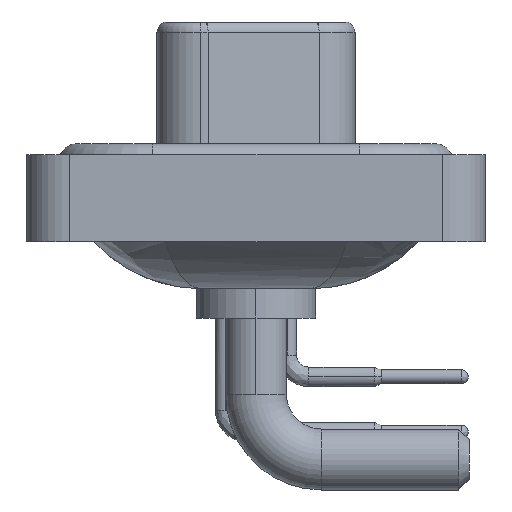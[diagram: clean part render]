
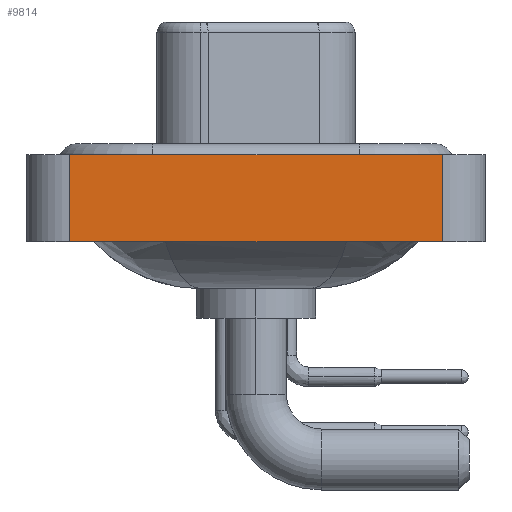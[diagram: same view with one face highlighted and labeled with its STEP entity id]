
A CAD part, left-side view. The second image highlights one B-rep face of the part: STEP entity #9814.
In plain terms, the highlighted planar face has unit normal (-1, 0, 0).
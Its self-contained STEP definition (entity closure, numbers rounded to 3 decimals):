
#1342 = CARTESIAN_POINT ( 'NONE',  ( -7.35, -8.55, 0.4 ) ) ;
#1466 = DIRECTION ( 'NONE',  ( 0., -1., 0. ) ) ;
#1738 = PLANE ( 'NONE',  #18898 ) ;
#3539 = DIRECTION ( 'NONE',  ( -1., 0., 0. ) ) ;
#3725 = EDGE_CURVE ( 'NONE', #19844, #24906, #16685, .T. ) ;
#3857 = DIRECTION ( 'NONE',  ( 0., 0., 1. ) ) ;
#4810 = ORIENTED_EDGE ( 'NONE', *, *, #3725, .F. ) ;
#5682 = CARTESIAN_POINT ( 'NONE',  ( -7.35, 8.55, -3.6 ) ) ;
#5730 = DIRECTION ( 'NONE',  ( 0., -1., 0. ) ) ;
#7687 = FACE_OUTER_BOUND ( 'NONE', #8082, .T. ) ;
#7811 = CARTESIAN_POINT ( 'NONE',  ( -7.35, -8.55, -3.6 ) ) ;
#8082 = EDGE_LOOP ( 'NONE', ( #26727, #4810, #15381, #11555 ) ) ;
#8461 = CARTESIAN_POINT ( 'NONE',  ( -7.35, -8.55, -3.6 ) ) ;
#9669 = VECTOR ( 'NONE', #24639, 1000. ) ;
#9814 = ADVANCED_FACE ( 'NONE', ( #7687 ), #1738, .T. ) ;
#10704 = EDGE_CURVE ( 'NONE', #17565, #19844, #15774, .T. ) ;
#11298 = EDGE_CURVE ( 'NONE', #12120, #24906, #16441, .T. ) ;
#11555 = ORIENTED_EDGE ( 'NONE', *, *, #19755, .T. ) ;
#12120 = VERTEX_POINT ( 'NONE', #8461 ) ;
#14320 = CARTESIAN_POINT ( 'NONE',  ( -7.35, -8.55, -3.6 ) ) ;
#15381 = ORIENTED_EDGE ( 'NONE', *, *, #10704, .F. ) ;
#15774 = LINE ( 'NONE', #5682, #9669 ) ;
#15986 = VECTOR ( 'NONE', #1466, 1000. ) ;
#16101 = LINE ( 'NONE', #7811, #23986 ) ;
#16441 = LINE ( 'NONE', #22824, #27150 ) ;
#16685 = LINE ( 'NONE', #20277, #15986 ) ;
#17565 = VERTEX_POINT ( 'NONE', #19744 ) ;
#18334 = CARTESIAN_POINT ( 'NONE',  ( -7.35, 8.55, 0.4 ) ) ;
#18898 = AXIS2_PLACEMENT_3D ( 'NONE', #14320, #3539, #27047 ) ;
#19744 = CARTESIAN_POINT ( 'NONE',  ( -7.35, 8.55, -3.6 ) ) ;
#19755 = EDGE_CURVE ( 'NONE', #17565, #12120, #16101, .T. ) ;
#19844 = VERTEX_POINT ( 'NONE', #18334 ) ;
#20277 = CARTESIAN_POINT ( 'NONE',  ( -7.35, -8.55, 0.4 ) ) ;
#22824 = CARTESIAN_POINT ( 'NONE',  ( -7.35, -8.55, -3.6 ) ) ;
#23986 = VECTOR ( 'NONE', #5730, 1000. ) ;
#24639 = DIRECTION ( 'NONE',  ( 0., 0., 1. ) ) ;
#24906 = VERTEX_POINT ( 'NONE', #1342 ) ;
#26727 = ORIENTED_EDGE ( 'NONE', *, *, #11298, .T. ) ;
#27047 = DIRECTION ( 'NONE',  ( 0., 0., 1. ) ) ;
#27150 = VECTOR ( 'NONE', #3857, 1000. ) ;
